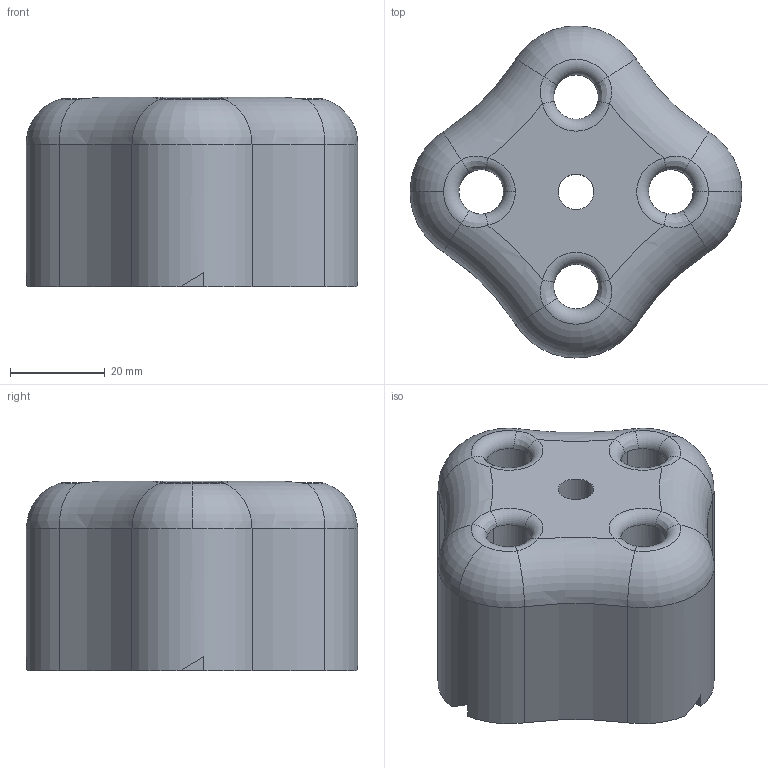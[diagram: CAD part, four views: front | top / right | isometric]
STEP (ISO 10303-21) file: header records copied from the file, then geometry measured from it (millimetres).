
FILE_DESCRIPTION (( 'STEP AP203' ), '1' );
FILE_NAME ('Barrel.STEP', '2013-11-14T05:10:01', ( '' ), ( '' ), 'SwSTEP 2.0', 'SolidWorks 2013', '' );
FILE_SCHEMA (( 'CONFIG_CONTROL_DESIGN' ));
Length unit declared in the file: millimetre
Products named in the file (1): Barrel
Bounding box: 70 x 70 x 40 mm (x, y, z)
Volume: 106059.1 mm3; surface area: 18660.2 mm2
Topology: 1 solids, 1 shells, 80 faces, 201 edges, 123 vertices
Faces by surface type: torus 28, cylinder 26, plane 18, bspline 8
Entity records: 2877 total; most frequent: CARTESIAN_POINT 857, DIRECTION 438, ORIENTED_EDGE 402, EDGE_CURVE 201, AXIS2_PLACEMENT_3D 192, VERTEX_POINT 123, CIRCLE 119, EDGE_LOOP 90
